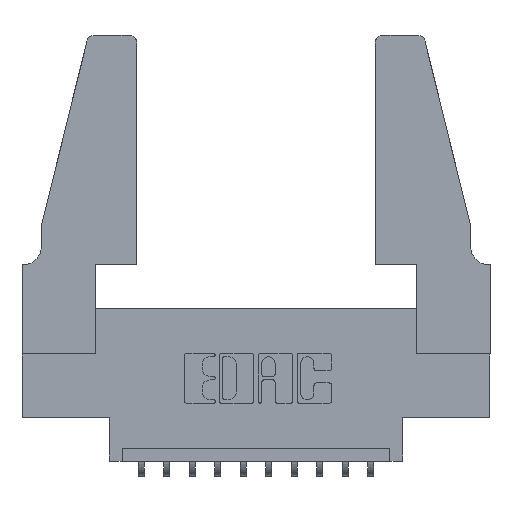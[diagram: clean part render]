
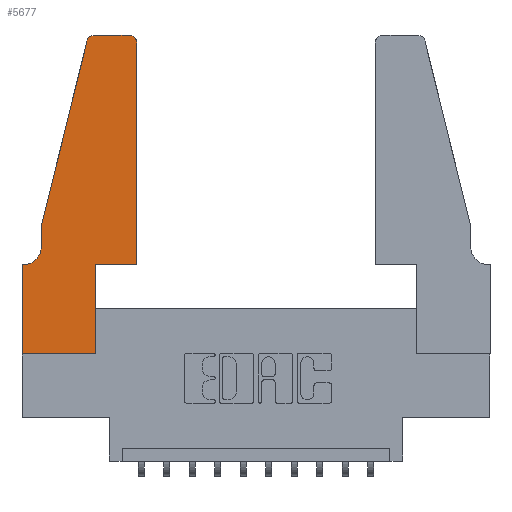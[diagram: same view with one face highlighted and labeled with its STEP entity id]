
A CAD part, top view. The second image highlights one B-rep face of the part: STEP entity #5677.
In plain terms, the highlighted planar face has unit normal (0, 0, 1).
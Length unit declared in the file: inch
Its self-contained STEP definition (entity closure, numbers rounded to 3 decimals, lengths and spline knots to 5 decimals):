
#28 = CARTESIAN_POINT ( 'NONE',  ( 0.4505, 1.22, 0.37 ) ) ;
#251 = ORIENTED_EDGE ( 'NONE', *, *, #5029, .T. ) ;
#407 = DIRECTION ( 'NONE',  ( 0., 0., 1. ) ) ;
#673 = VECTOR ( 'NONE', #920, 39.37008 ) ;
#920 = DIRECTION ( 'NONE',  ( 0., 1., 0. ) ) ;
#1053 = VERTEX_POINT ( 'NONE', #10790 ) ;
#1151 = VERTEX_POINT ( 'NONE', #28 ) ;
#1164 = CIRCLE ( 'NONE', #7050, 0.03 ) ;
#1196 = VERTEX_POINT ( 'NONE', #10110 ) ;
#1233 = VERTEX_POINT ( 'NONE', #13786 ) ;
#1293 = ORIENTED_EDGE ( 'NONE', *, *, #7524, .T. ) ;
#1499 = FACE_OUTER_BOUND ( 'NONE', #3715, .T. ) ;
#1710 = ORIENTED_EDGE ( 'NONE', *, *, #3934, .T. ) ;
#1768 = CARTESIAN_POINT ( 'NONE',  ( 0.2865, 0.35, 0.37 ) ) ;
#1791 = CARTESIAN_POINT ( 'NONE',  ( 0., 0., 0.37 ) ) ;
#2044 = CARTESIAN_POINT ( 'NONE',  ( 0.4505, 0.35, 0.37 ) ) ;
#2173 = LINE ( 'NONE', #1791, #7324 ) ;
#2299 = ORIENTED_EDGE ( 'NONE', *, *, #8624, .T. ) ;
#2411 = VECTOR ( 'NONE', #10818, 39.37008 ) ;
#2486 = EDGE_CURVE ( 'NONE', #3647, #11880, #10522, .T. ) ;
#2911 = PLANE ( 'NONE',  #12003 ) ;
#3099 = CARTESIAN_POINT ( 'NONE',  ( 0.284, 1.22, 0.37 ) ) ;
#3299 = DIRECTION ( 'NONE',  ( -1., 0., 0. ) ) ;
#3382 = VERTEX_POINT ( 'NONE', #4879 ) ;
#3647 = VERTEX_POINT ( 'NONE', #8064 ) ;
#3715 = EDGE_LOOP ( 'NONE', ( #5765, #251, #1293, #4783, #10561, #1710, #7977, #4053, #11814, #2299, #10401, #11669 ) ) ;
#3740 = DIRECTION ( 'NONE',  ( 0., 0., 1. ) ) ;
#3880 = CARTESIAN_POINT ( 'NONE',  ( 0., 0., 0.37 ) ) ;
#3934 = EDGE_CURVE ( 'NONE', #3382, #1196, #13047, .T. ) ;
#3954 = DIRECTION ( 'NONE',  ( 0., 1., 0. ) ) ;
#4051 = EDGE_CURVE ( 'NONE', #1053, #1151, #5668, .T. ) ;
#4053 = ORIENTED_EDGE ( 'NONE', *, *, #12626, .T. ) ;
#4057 = CIRCLE ( 'NONE', #4887, 0.03 ) ;
#4471 = DIRECTION ( 'NONE',  ( -1., 0., 0. ) ) ;
#4783 = ORIENTED_EDGE ( 'NONE', *, *, #2486, .T. ) ;
#4879 = CARTESIAN_POINT ( 'NONE',  ( 0.0055, 0.35, 0.37 ) ) ;
#4887 = AXIS2_PLACEMENT_3D ( 'NONE', #12472, #407, #13648 ) ;
#5029 = EDGE_CURVE ( 'NONE', #6902, #10265, #1164, .T. ) ;
#5093 = EDGE_CURVE ( 'NONE', #11880, #3382, #9047, .T. ) ;
#5621 = LINE ( 'NONE', #10611, #9905 ) ;
#5640 = CARTESIAN_POINT ( 'NONE',  ( 0.2865, 0., 0.37 ) ) ;
#5668 = LINE ( 'NONE', #2044, #673 ) ;
#5677 = ADVANCED_FACE ( 'NONE', ( #1499 ), #2911, .T. ) ;
#5765 = ORIENTED_EDGE ( 'NONE', *, *, #12254, .T. ) ;
#5767 = CARTESIAN_POINT ( 'NONE',  ( 0.0755, 0.42, 0.37 ) ) ;
#5930 = CARTESIAN_POINT ( 'NONE',  ( 0.25487, 1.22718, 0.37 ) ) ;
#6052 = EDGE_CURVE ( 'NONE', #1196, #1233, #2173, .T. ) ;
#6092 = LINE ( 'NONE', #6390, #11225 ) ;
#6390 = CARTESIAN_POINT ( 'NONE',  ( 0.0755, 0.5, 0.37 ) ) ;
#6649 = CARTESIAN_POINT ( 'NONE',  ( 0.0055, 0.42, 0.37 ) ) ;
#6902 = VERTEX_POINT ( 'NONE', #13601 ) ;
#7050 = AXIS2_PLACEMENT_3D ( 'NONE', #3099, #10621, #11742 ) ;
#7324 = VECTOR ( 'NONE', #9408, 39.37008 ) ;
#7524 = EDGE_CURVE ( 'NONE', #10265, #3647, #6092, .T. ) ;
#7573 = VECTOR ( 'NONE', #12006, 39.37008 ) ;
#7977 = ORIENTED_EDGE ( 'NONE', *, *, #6052, .T. ) ;
#8064 = CARTESIAN_POINT ( 'NONE',  ( 0.0755, 0.5, 0.37 ) ) ;
#8157 = LINE ( 'NONE', #1768, #10049 ) ;
#8559 = VERTEX_POINT ( 'NONE', #12711 ) ;
#8588 = DIRECTION ( 'NONE',  ( -0.239, -0.971, 0. ) ) ;
#8624 = EDGE_CURVE ( 'NONE', #8559, #1053, #5621, .T. ) ;
#8774 = AXIS2_PLACEMENT_3D ( 'NONE', #6649, #14203, #3299 ) ;
#9047 = CIRCLE ( 'NONE', #8774, 0.07 ) ;
#9408 = DIRECTION ( 'NONE',  ( 0., -1., 0. ) ) ;
#9420 = EDGE_CURVE ( 'NONE', #12079, #8559, #8157, .T. ) ;
#9477 = CARTESIAN_POINT ( 'NONE',  ( 0.0755, 0.5, 0.37 ) ) ;
#9618 = DIRECTION ( 'NONE',  ( 0., -1., 0. ) ) ;
#9661 = CARTESIAN_POINT ( 'NONE',  ( 0.0755, 0.35, 0.37 ) ) ;
#9905 = VECTOR ( 'NONE', #12822, 39.37008 ) ;
#10049 = VECTOR ( 'NONE', #3954, 39.37008 ) ;
#10110 = CARTESIAN_POINT ( 'NONE',  ( 0., 0.35, 0.37 ) ) ;
#10146 = EDGE_CURVE ( 'NONE', #1151, #10578, #4057, .T. ) ;
#10265 = VERTEX_POINT ( 'NONE', #5930 ) ;
#10401 = ORIENTED_EDGE ( 'NONE', *, *, #4051, .T. ) ;
#10498 = LINE ( 'NONE', #3880, #7573 ) ;
#10522 = LINE ( 'NONE', #9477, #11575 ) ;
#10561 = ORIENTED_EDGE ( 'NONE', *, *, #5093, .T. ) ;
#10578 = VERTEX_POINT ( 'NONE', #12102 ) ;
#10611 = CARTESIAN_POINT ( 'NONE',  ( 0.4505, 0.35, 0.37 ) ) ;
#10621 = DIRECTION ( 'NONE',  ( 0., 0., 1. ) ) ;
#10625 = CARTESIAN_POINT ( 'NONE',  ( 0., 0.35, 0.37 ) ) ;
#10790 = CARTESIAN_POINT ( 'NONE',  ( 0.4505, 0.35, 0.37 ) ) ;
#10818 = DIRECTION ( 'NONE',  ( -1., 0., 0. ) ) ;
#11008 = LINE ( 'NONE', #11015, #11381 ) ;
#11015 = CARTESIAN_POINT ( 'NONE',  ( 0.2605, 1.25, 0.37 ) ) ;
#11225 = VECTOR ( 'NONE', #8588, 39.37008 ) ;
#11381 = VECTOR ( 'NONE', #4471, 39.37008 ) ;
#11493 = DIRECTION ( 'NONE',  ( 1., 0., 0. ) ) ;
#11575 = VECTOR ( 'NONE', #9618, 39.37008 ) ;
#11669 = ORIENTED_EDGE ( 'NONE', *, *, #10146, .T. ) ;
#11742 = DIRECTION ( 'NONE',  ( 1., 0., 0. ) ) ;
#11814 = ORIENTED_EDGE ( 'NONE', *, *, #9420, .T. ) ;
#11880 = VERTEX_POINT ( 'NONE', #5767 ) ;
#12003 = AXIS2_PLACEMENT_3D ( 'NONE', #10625, #3740, #11493 ) ;
#12006 = DIRECTION ( 'NONE',  ( 1., 0., 0. ) ) ;
#12079 = VERTEX_POINT ( 'NONE', #5640 ) ;
#12102 = CARTESIAN_POINT ( 'NONE',  ( 0.4205, 1.25, 0.37 ) ) ;
#12254 = EDGE_CURVE ( 'NONE', #10578, #6902, #11008, .T. ) ;
#12472 = CARTESIAN_POINT ( 'NONE',  ( 0.4205, 1.22, 0.37 ) ) ;
#12626 = EDGE_CURVE ( 'NONE', #1233, #12079, #10498, .T. ) ;
#12711 = CARTESIAN_POINT ( 'NONE',  ( 0.2865, 0.35, 0.37 ) ) ;
#12822 = DIRECTION ( 'NONE',  ( 1., 0., 0. ) ) ;
#13047 = LINE ( 'NONE', #9661, #2411 ) ;
#13601 = CARTESIAN_POINT ( 'NONE',  ( 0.284, 1.25, 0.37 ) ) ;
#13648 = DIRECTION ( 'NONE',  ( 1., 0., 0. ) ) ;
#13786 = CARTESIAN_POINT ( 'NONE',  ( 0., 0., 0.37 ) ) ;
#14203 = DIRECTION ( 'NONE',  ( 0., 0., -1. ) ) ;
